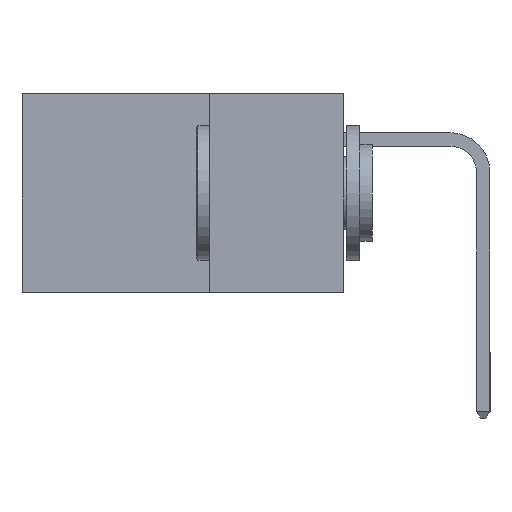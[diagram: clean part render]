
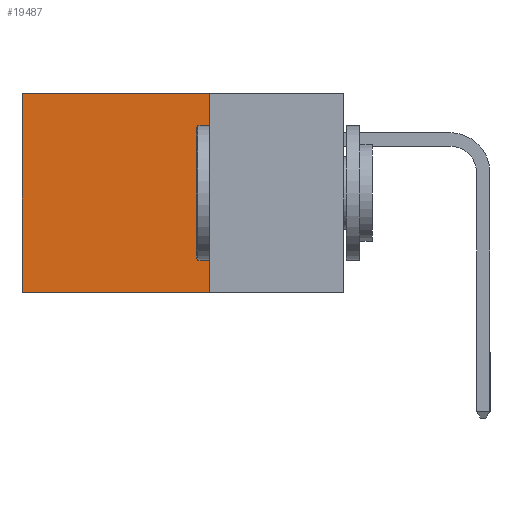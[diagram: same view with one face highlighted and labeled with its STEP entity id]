
A CAD part, left-side view. The second image highlights one B-rep face of the part: STEP entity #19487.
In plain terms, the highlighted planar face has unit normal (-1, 0, 0).
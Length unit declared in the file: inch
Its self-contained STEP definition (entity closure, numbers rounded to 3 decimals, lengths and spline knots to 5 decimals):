
#102 = ORIENTED_EDGE ( 'NONE', *, *, #12015, .F. ) ;
#178 = EDGE_CURVE ( 'NONE', #24831, #27000, #18040, .T. ) ;
#221 = DIRECTION ( 'NONE',  ( 0., 1., 0. ) ) ;
#981 = DIRECTION ( 'NONE',  ( 0., 0., -1. ) ) ;
#2192 = LINE ( 'NONE', #17908, #14494 ) ;
#2614 = EDGE_CURVE ( 'NONE', #24831, #9737, #2192, .T. ) ;
#4368 = CARTESIAN_POINT ( 'NONE',  ( 0.298, 0.6, -0.37 ) ) ;
#4472 = CARTESIAN_POINT ( 'NONE',  ( 0.298, 0.25, 0. ) ) ;
#4508 = CARTESIAN_POINT ( 'NONE',  ( 0.298, 0.6, 0. ) ) ;
#4681 = VECTOR ( 'NONE', #221, 39.37008 ) ;
#7500 = VERTEX_POINT ( 'NONE', #4368 ) ;
#8580 = PLANE ( 'NONE',  #18837 ) ;
#8980 = EDGE_LOOP ( 'NONE', ( #21819, #102, #25746, #23671 ) ) ;
#9737 = VERTEX_POINT ( 'NONE', #10360 ) ;
#10360 = CARTESIAN_POINT ( 'NONE',  ( 0.298, 0.25, -0.37 ) ) ;
#12015 = EDGE_CURVE ( 'NONE', #9737, #7500, #14813, .T. ) ;
#12891 = CARTESIAN_POINT ( 'NONE',  ( 0.298, 0.25, 0. ) ) ;
#13267 = DIRECTION ( 'NONE',  ( 0., 0., -1. ) ) ;
#14494 = VECTOR ( 'NONE', #981, 39.37008 ) ;
#14813 = LINE ( 'NONE', #16060, #25066 ) ;
#16060 = CARTESIAN_POINT ( 'NONE',  ( 0.298, 0.25, -0.37 ) ) ;
#16682 = VECTOR ( 'NONE', #23835, 39.37008 ) ;
#17908 = CARTESIAN_POINT ( 'NONE',  ( 0.298, 0.25, 0. ) ) ;
#18040 = LINE ( 'NONE', #4472, #4681 ) ;
#18086 = DIRECTION ( 'NONE',  ( 0., 1., 0. ) ) ;
#18837 = AXIS2_PLACEMENT_3D ( 'NONE', #12891, #28166, #13267 ) ;
#19487 = ADVANCED_FACE ( 'NONE', ( #22378 ), #8580, .F. ) ;
#20892 = EDGE_CURVE ( 'NONE', #27000, #7500, #26953, .T. ) ;
#21819 = ORIENTED_EDGE ( 'NONE', *, *, #20892, .T. ) ;
#22036 = CARTESIAN_POINT ( 'NONE',  ( 0.298, 0.25, 0. ) ) ;
#22378 = FACE_OUTER_BOUND ( 'NONE', #8980, .T. ) ;
#23671 = ORIENTED_EDGE ( 'NONE', *, *, #178, .T. ) ;
#23835 = DIRECTION ( 'NONE',  ( 0., 0., -1. ) ) ;
#24831 = VERTEX_POINT ( 'NONE', #22036 ) ;
#25066 = VECTOR ( 'NONE', #18086, 39.37008 ) ;
#25158 = CARTESIAN_POINT ( 'NONE',  ( 0.298, 0.6, 0. ) ) ;
#25746 = ORIENTED_EDGE ( 'NONE', *, *, #2614, .F. ) ;
#26953 = LINE ( 'NONE', #4508, #16682 ) ;
#27000 = VERTEX_POINT ( 'NONE', #25158 ) ;
#28166 = DIRECTION ( 'NONE',  ( 1., 0., 0. ) ) ;
